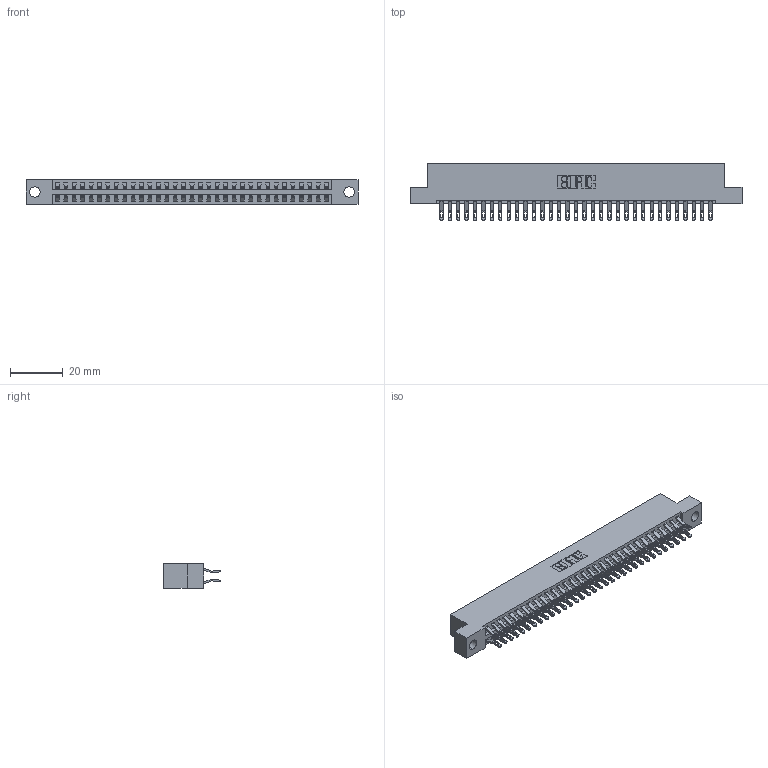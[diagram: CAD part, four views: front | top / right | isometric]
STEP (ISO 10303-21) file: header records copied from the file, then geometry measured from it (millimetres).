
FILE_DESCRIPTION (( 'STEP AP203' ), '1' );
FILE_NAME ('396-066-555-204.STEP', '2019-10-30T18:24:58', ( '' ), ( '' ), 'SwSTEP 2.0', 'SolidWorks 2016', '' );
FILE_SCHEMA (( 'CONFIG_CONTROL_DESIGN' ));
Length unit declared in the file: inch
Products named in the file (3): 346 Part_Flush Mounting Lugs - 0.156 Dia-TH; 345-292-001_555 Tail; 396-066-555-204
Assembly tree (67 placements, depth 2):
  396-066-555-204
    346 Part_Flush Mounting Lugs - 0.156 Dia-TH
    345-292-001_555 Tail  x66
Bounding box: 125.35 x 21.46 x 9.4 mm (x, y, z)
Volume: 12256.8 mm3; surface area: 17202 mm2
Topology: 67 solids, 67 shells, 3950 faces, 12407 edges, 8270 vertices
Faces by surface type: plane 2254, cylinder 1696
Entity records: 23077 total; most frequent: CARTESIAN_POINT 3850, ORIENTED_EDGE 3754, DIRECTION 3413, EDGE_CURVE 1877, VECTOR 1593, LINE 1593, VERTEX_POINT 1250, AXIS2_PLACEMENT_3D 910
